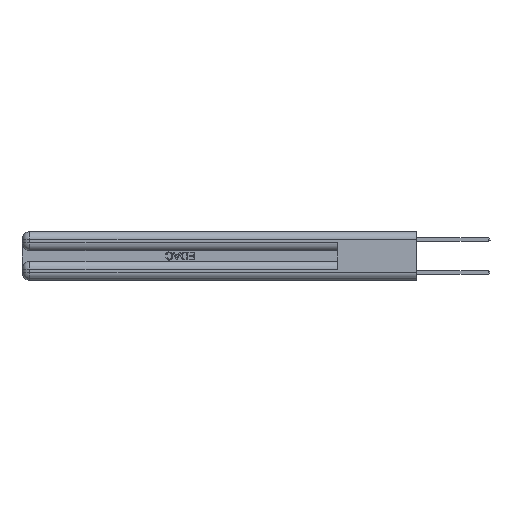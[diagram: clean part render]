
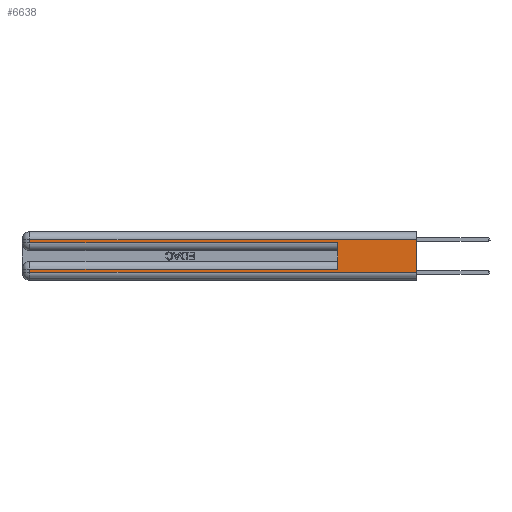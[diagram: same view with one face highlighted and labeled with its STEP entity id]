
A CAD part, left-side view. The second image highlights one B-rep face of the part: STEP entity #6638.
In plain terms, the highlighted planar face has unit normal (-1, 0, 0).
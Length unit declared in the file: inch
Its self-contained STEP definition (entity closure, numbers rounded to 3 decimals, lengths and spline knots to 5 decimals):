
#64 = EDGE_CURVE ( 'NONE', #3769, #21326, #29233, .T. ) ;
#938 = EDGE_CURVE ( 'NONE', #7189, #17158, #19143, .T. ) ;
#1616 = VECTOR ( 'NONE', #22054, 39.37008 ) ;
#1679 = ORIENTED_EDGE ( 'NONE', *, *, #11387, .T. ) ;
#2082 = CARTESIAN_POINT ( 'NONE',  ( 0., 2.94, 0.285 ) ) ;
#2415 = VECTOR ( 'NONE', #18688, 39.37008 ) ;
#3425 = LINE ( 'NONE', #13258, #18189 ) ;
#3769 = VERTEX_POINT ( 'NONE', #7385 ) ;
#4468 = CARTESIAN_POINT ( 'NONE',  ( 0., 0., 0.31 ) ) ;
#4714 = CARTESIAN_POINT ( 'NONE',  ( 0., 0., 0.06 ) ) ;
#6638 = ADVANCED_FACE ( 'NONE', ( #25894 ), #14605, .F. ) ;
#6993 = DIRECTION ( 'NONE',  ( 0., 0., -1. ) ) ;
#7011 = CARTESIAN_POINT ( 'NONE',  ( 0., 0., 0.085 ) ) ;
#7189 = VERTEX_POINT ( 'NONE', #11051 ) ;
#7336 = EDGE_CURVE ( 'NONE', #15015, #17158, #3425, .T. ) ;
#7385 = CARTESIAN_POINT ( 'NONE',  ( 0., 2.94, 0.31 ) ) ;
#8630 = CARTESIAN_POINT ( 'NONE',  ( 0., 2.94, 0.37 ) ) ;
#9474 = CARTESIAN_POINT ( 'NONE',  ( 0., 0.6, 0.085 ) ) ;
#10604 = EDGE_CURVE ( 'NONE', #15015, #3769, #29634, .T. ) ;
#10714 = CARTESIAN_POINT ( 'NONE',  ( 0., 0.6, 0.145 ) ) ;
#11051 = CARTESIAN_POINT ( 'NONE',  ( 0., 2.94, 0.06 ) ) ;
#11056 = DIRECTION ( 'NONE',  ( 0., 0., 1. ) ) ;
#11387 = EDGE_CURVE ( 'NONE', #28882, #7189, #18221, .T. ) ;
#12597 = CARTESIAN_POINT ( 'NONE',  ( 0., 0.6, 0.285 ) ) ;
#12820 = LINE ( 'NONE', #7011, #1616 ) ;
#13258 = CARTESIAN_POINT ( 'NONE',  ( 0., 0., 0.37 ) ) ;
#13703 = ORIENTED_EDGE ( 'NONE', *, *, #938, .T. ) ;
#14605 = PLANE ( 'NONE',  #18494 ) ;
#15015 = VERTEX_POINT ( 'NONE', #4468 ) ;
#15270 = DIRECTION ( 'NONE',  ( 0., -1., 0. ) ) ;
#15638 = DIRECTION ( 'NONE',  ( 0., 0., -1. ) ) ;
#15686 = CARTESIAN_POINT ( 'NONE',  ( 0., 0., 0.285 ) ) ;
#17158 = VERTEX_POINT ( 'NONE', #4714 ) ;
#17441 = VECTOR ( 'NONE', #11056, 39.37008 ) ;
#17488 = ORIENTED_EDGE ( 'NONE', *, *, #21037, .F. ) ;
#17988 = VECTOR ( 'NONE', #6993, 39.37008 ) ;
#18014 = DIRECTION ( 'NONE',  ( 0., 0., -1. ) ) ;
#18122 = DIRECTION ( 'NONE',  ( 0., -1., 0. ) ) ;
#18189 = VECTOR ( 'NONE', #18014, 39.37008 ) ;
#18221 = LINE ( 'NONE', #8630, #23093 ) ;
#18494 = AXIS2_PLACEMENT_3D ( 'NONE', #22442, #24903, #27585 ) ;
#18688 = DIRECTION ( 'NONE',  ( 0., 1., 0. ) ) ;
#18815 = CARTESIAN_POINT ( 'NONE',  ( 0., 0., 0.31 ) ) ;
#19065 = LINE ( 'NONE', #10714, #17441 ) ;
#19143 = LINE ( 'NONE', #26615, #25172 ) ;
#21037 = EDGE_CURVE ( 'NONE', #26943, #21303, #19065, .T. ) ;
#21303 = VERTEX_POINT ( 'NONE', #12597 ) ;
#21326 = VERTEX_POINT ( 'NONE', #2082 ) ;
#21458 = EDGE_CURVE ( 'NONE', #21326, #21303, #30633, .T. ) ;
#22054 = DIRECTION ( 'NONE',  ( 0., 1., 0. ) ) ;
#22256 = CARTESIAN_POINT ( 'NONE',  ( 0., 2.94, 0.37 ) ) ;
#22442 = CARTESIAN_POINT ( 'NONE',  ( 0., 0., 0.37 ) ) ;
#23093 = VECTOR ( 'NONE', #15638, 39.37008 ) ;
#24903 = DIRECTION ( 'NONE',  ( 1., 0., 0. ) ) ;
#25133 = CARTESIAN_POINT ( 'NONE',  ( 0., 2.94, 0.085 ) ) ;
#25172 = VECTOR ( 'NONE', #15270, 39.37008 ) ;
#25894 = FACE_OUTER_BOUND ( 'NONE', #29490, .T. ) ;
#26615 = CARTESIAN_POINT ( 'NONE',  ( 0., 0., 0.06 ) ) ;
#26943 = VERTEX_POINT ( 'NONE', #9474 ) ;
#27243 = ORIENTED_EDGE ( 'NONE', *, *, #32479, .T. ) ;
#27585 = DIRECTION ( 'NONE',  ( 0., 0., -1. ) ) ;
#28668 = ORIENTED_EDGE ( 'NONE', *, *, #7336, .F. ) ;
#28882 = VERTEX_POINT ( 'NONE', #25133 ) ;
#29233 = LINE ( 'NONE', #22256, #17988 ) ;
#29490 = EDGE_LOOP ( 'NONE', ( #28668, #31539, #33078, #30219, #17488, #27243, #1679, #13703 ) ) ;
#29634 = LINE ( 'NONE', #18815, #2415 ) ;
#30219 = ORIENTED_EDGE ( 'NONE', *, *, #21458, .T. ) ;
#30633 = LINE ( 'NONE', #15686, #32659 ) ;
#31539 = ORIENTED_EDGE ( 'NONE', *, *, #10604, .T. ) ;
#32479 = EDGE_CURVE ( 'NONE', #26943, #28882, #12820, .T. ) ;
#32659 = VECTOR ( 'NONE', #18122, 39.37008 ) ;
#33078 = ORIENTED_EDGE ( 'NONE', *, *, #64, .T. ) ;
